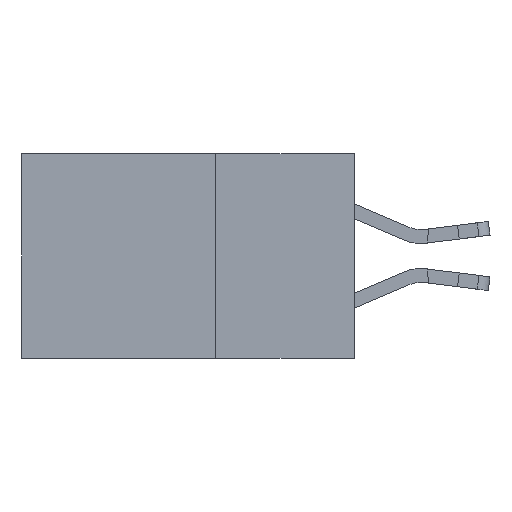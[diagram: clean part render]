
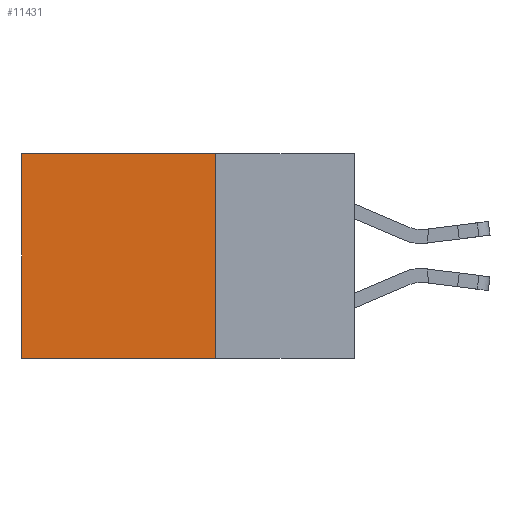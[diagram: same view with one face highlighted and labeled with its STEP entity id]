
A CAD part, left-side view. The second image highlights one B-rep face of the part: STEP entity #11431.
In plain terms, the highlighted planar face has unit normal (-1, 0, 0).
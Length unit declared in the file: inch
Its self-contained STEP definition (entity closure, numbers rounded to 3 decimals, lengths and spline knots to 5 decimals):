
#123 = ORIENTED_EDGE ( 'NONE', *, *, #8853, .T. ) ;
#315 = AXIS2_PLACEMENT_3D ( 'NONE', #8053, #9054, #3185 ) ;
#507 = DIRECTION ( 'NONE',  ( 0., 1., 0. ) ) ;
#990 = CARTESIAN_POINT ( 'NONE',  ( 0.298, 0.25, 0. ) ) ;
#1202 = CARTESIAN_POINT ( 'NONE',  ( 0.298, 0.25, -0.37 ) ) ;
#1358 = ORIENTED_EDGE ( 'NONE', *, *, #7434, .F. ) ;
#2095 = VERTEX_POINT ( 'NONE', #3003 ) ;
#2496 = LINE ( 'NONE', #5438, #12610 ) ;
#2608 = CARTESIAN_POINT ( 'NONE',  ( 0.298, 0.6, 0. ) ) ;
#3003 = CARTESIAN_POINT ( 'NONE',  ( 0.298, 0.25, 0. ) ) ;
#3185 = DIRECTION ( 'NONE',  ( 0., 0., -1. ) ) ;
#3898 = VERTEX_POINT ( 'NONE', #8550 ) ;
#4300 = LINE ( 'NONE', #990, #5932 ) ;
#4539 = EDGE_CURVE ( 'NONE', #3898, #11694, #7615, .T. ) ;
#4604 = DIRECTION ( 'NONE',  ( 0., 0., -1. ) ) ;
#4965 = EDGE_LOOP ( 'NONE', ( #10796, #1358, #5470, #123 ) ) ;
#5013 = VECTOR ( 'NONE', #10464, 39.37008 ) ;
#5438 = CARTESIAN_POINT ( 'NONE',  ( 0.298, 0.25, -0.37 ) ) ;
#5470 = ORIENTED_EDGE ( 'NONE', *, *, #8618, .F. ) ;
#5932 = VECTOR ( 'NONE', #7882, 39.37008 ) ;
#6264 = LINE ( 'NONE', #10481, #6585 ) ;
#6585 = VECTOR ( 'NONE', #4604, 39.37008 ) ;
#7248 = VERTEX_POINT ( 'NONE', #1202 ) ;
#7434 = EDGE_CURVE ( 'NONE', #7248, #11694, #2496, .T. ) ;
#7510 = CARTESIAN_POINT ( 'NONE',  ( 0.298, 0.6, -0.37 ) ) ;
#7583 = FACE_OUTER_BOUND ( 'NONE', #4965, .T. ) ;
#7615 = LINE ( 'NONE', #2608, #5013 ) ;
#7882 = DIRECTION ( 'NONE',  ( 0., 1., 0. ) ) ;
#8053 = CARTESIAN_POINT ( 'NONE',  ( 0.298, 0.25, 0. ) ) ;
#8550 = CARTESIAN_POINT ( 'NONE',  ( 0.298, 0.6, 0. ) ) ;
#8618 = EDGE_CURVE ( 'NONE', #2095, #7248, #6264, .T. ) ;
#8853 = EDGE_CURVE ( 'NONE', #2095, #3898, #4300, .T. ) ;
#9054 = DIRECTION ( 'NONE',  ( 1., 0., 0. ) ) ;
#10464 = DIRECTION ( 'NONE',  ( 0., 0., -1. ) ) ;
#10481 = CARTESIAN_POINT ( 'NONE',  ( 0.298, 0.25, 0. ) ) ;
#10796 = ORIENTED_EDGE ( 'NONE', *, *, #4539, .T. ) ;
#10984 = PLANE ( 'NONE',  #315 ) ;
#11431 = ADVANCED_FACE ( 'NONE', ( #7583 ), #10984, .F. ) ;
#11694 = VERTEX_POINT ( 'NONE', #7510 ) ;
#12610 = VECTOR ( 'NONE', #507, 39.37008 ) ;
